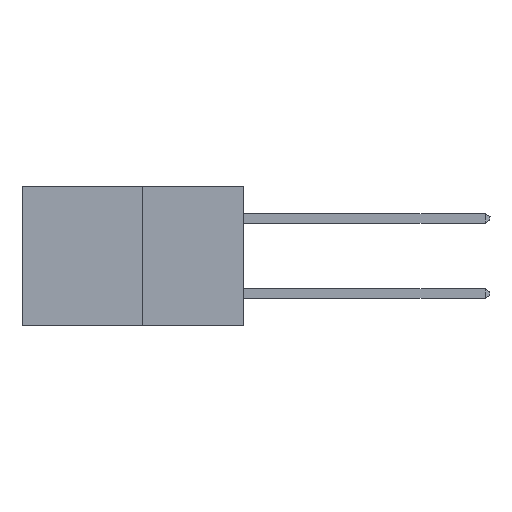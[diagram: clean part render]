
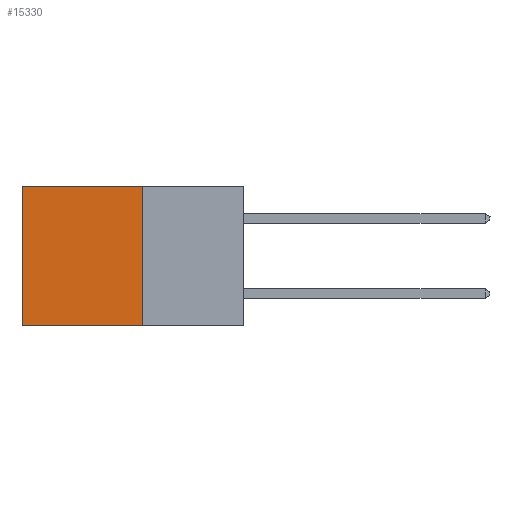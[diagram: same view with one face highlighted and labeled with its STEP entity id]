
A CAD part, left-side view. The second image highlights one B-rep face of the part: STEP entity #15330.
In plain terms, the highlighted planar face has unit normal (-1, 0, 0).
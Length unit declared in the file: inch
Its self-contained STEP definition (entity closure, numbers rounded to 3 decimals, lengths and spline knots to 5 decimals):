
#1038 = VERTEX_POINT ( 'NONE', #8170 ) ;
#2791 = LINE ( 'NONE', #25104, #14772 ) ;
#5774 = VECTOR ( 'NONE', #8902, 39.37008 ) ;
#6037 = LINE ( 'NONE', #18171, #22766 ) ;
#7757 = DIRECTION ( 'NONE',  ( 0., 1., 0. ) ) ;
#8170 = CARTESIAN_POINT ( 'NONE',  ( 0.277, 0.59, 0. ) ) ;
#8315 = FACE_OUTER_BOUND ( 'NONE', #18201, .T. ) ;
#8902 = DIRECTION ( 'NONE',  ( 0., 0., -1. ) ) ;
#9897 = LINE ( 'NONE', #21994, #23220 ) ;
#10336 = ORIENTED_EDGE ( 'NONE', *, *, #20259, .F. ) ;
#11001 = CARTESIAN_POINT ( 'NONE',  ( 0.277, 0.27, -0.37 ) ) ;
#11142 = DIRECTION ( 'NONE',  ( 0., 0., -1. ) ) ;
#12976 = CARTESIAN_POINT ( 'NONE',  ( 0.277, 0.27, 0. ) ) ;
#13404 = DIRECTION ( 'NONE',  ( 0., 0., -1. ) ) ;
#13737 = VERTEX_POINT ( 'NONE', #12976 ) ;
#14772 = VECTOR ( 'NONE', #27466, 39.37008 ) ;
#15302 = AXIS2_PLACEMENT_3D ( 'NONE', #11001, #27521, #13404 ) ;
#15330 = ADVANCED_FACE ( 'NONE', ( #8315 ), #25163, .F. ) ;
#18171 = CARTESIAN_POINT ( 'NONE',  ( 0.277, 0.27, -0.37 ) ) ;
#18201 = EDGE_LOOP ( 'NONE', ( #25489, #23329, #10336, #20821 ) ) ;
#18423 = LINE ( 'NONE', #25454, #5774 ) ;
#18632 = CARTESIAN_POINT ( 'NONE',  ( 0.277, 0.59, -0.37 ) ) ;
#20259 = EDGE_CURVE ( 'NONE', #13737, #20790, #6037, .T. ) ;
#20790 = VERTEX_POINT ( 'NONE', #24544 ) ;
#20821 = ORIENTED_EDGE ( 'NONE', *, *, #24972, .T. ) ;
#21090 = VERTEX_POINT ( 'NONE', #18632 ) ;
#21994 = CARTESIAN_POINT ( 'NONE',  ( 0.277, 0.27, 0. ) ) ;
#22766 = VECTOR ( 'NONE', #11142, 39.37008 ) ;
#23220 = VECTOR ( 'NONE', #7757, 39.37008 ) ;
#23329 = ORIENTED_EDGE ( 'NONE', *, *, #24574, .F. ) ;
#24544 = CARTESIAN_POINT ( 'NONE',  ( 0.277, 0.27, -0.37 ) ) ;
#24574 = EDGE_CURVE ( 'NONE', #20790, #21090, #2791, .T. ) ;
#24972 = EDGE_CURVE ( 'NONE', #13737, #1038, #9897, .T. ) ;
#25104 = CARTESIAN_POINT ( 'NONE',  ( 0.277, 0.27, -0.37 ) ) ;
#25163 = PLANE ( 'NONE',  #15302 ) ;
#25454 = CARTESIAN_POINT ( 'NONE',  ( 0.277, 0.59, -0.37 ) ) ;
#25489 = ORIENTED_EDGE ( 'NONE', *, *, #27283, .T. ) ;
#27283 = EDGE_CURVE ( 'NONE', #1038, #21090, #18423, .T. ) ;
#27466 = DIRECTION ( 'NONE',  ( 0., 1., 0. ) ) ;
#27521 = DIRECTION ( 'NONE',  ( 1., 0., 0. ) ) ;
